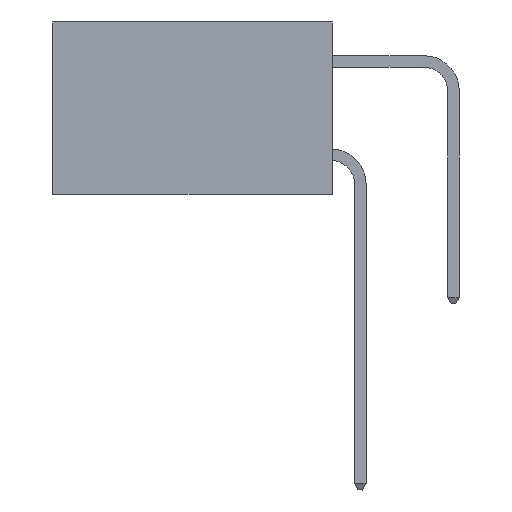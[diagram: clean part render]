
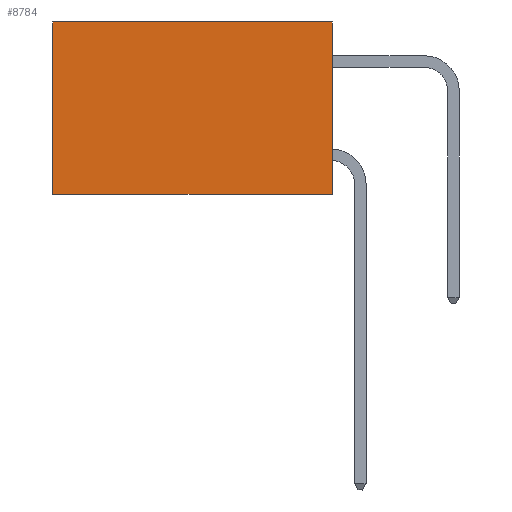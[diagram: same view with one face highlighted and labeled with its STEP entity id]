
A CAD part, left-side view. The second image highlights one B-rep face of the part: STEP entity #8784.
In plain terms, the highlighted planar face has unit normal (-1, 0, 0).
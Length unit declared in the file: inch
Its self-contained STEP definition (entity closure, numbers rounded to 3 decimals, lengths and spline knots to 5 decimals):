
#136 = FACE_OUTER_BOUND ( 'NONE', #17684, .T. ) ;
#1289 = VERTEX_POINT ( 'NONE', #6100 ) ;
#1593 = EDGE_CURVE ( 'NONE', #7111, #9854, #18074, .T. ) ;
#1920 = DIRECTION ( 'NONE',  ( 0., 1., 0. ) ) ;
#2348 = PLANE ( 'NONE',  #16039 ) ;
#2516 = EDGE_CURVE ( 'NONE', #5269, #1289, #4858, .T. ) ;
#4044 = CARTESIAN_POINT ( 'NONE',  ( 0.298, 0., -0.37 ) ) ;
#4463 = DIRECTION ( 'NONE',  ( 1., 0., 0. ) ) ;
#4858 = LINE ( 'NONE', #19780, #14758 ) ;
#4864 = CARTESIAN_POINT ( 'NONE',  ( 0.298, 0., 0. ) ) ;
#5269 = VERTEX_POINT ( 'NONE', #17595 ) ;
#6100 = CARTESIAN_POINT ( 'NONE',  ( 0.298, 0.6, 0. ) ) ;
#7111 = VERTEX_POINT ( 'NONE', #13817 ) ;
#7821 = VECTOR ( 'NONE', #18948, 39.37008 ) ;
#8350 = ORIENTED_EDGE ( 'NONE', *, *, #21593, .F. ) ;
#8784 = ADVANCED_FACE ( 'NONE', ( #136 ), #2348, .F. ) ;
#9854 = VERTEX_POINT ( 'NONE', #23760 ) ;
#12603 = EDGE_CURVE ( 'NONE', #1289, #9854, #21689, .T. ) ;
#13795 = VECTOR ( 'NONE', #1920, 39.37008 ) ;
#13817 = CARTESIAN_POINT ( 'NONE',  ( 0.298, 0., -0.37 ) ) ;
#14229 = ORIENTED_EDGE ( 'NONE', *, *, #2516, .T. ) ;
#14758 = VECTOR ( 'NONE', #23289, 39.37008 ) ;
#16039 = AXIS2_PLACEMENT_3D ( 'NONE', #22189, #4463, #20253 ) ;
#16860 = ORIENTED_EDGE ( 'NONE', *, *, #1593, .F. ) ;
#17594 = VECTOR ( 'NONE', #20561, 39.37008 ) ;
#17595 = CARTESIAN_POINT ( 'NONE',  ( 0.298, 0., 0. ) ) ;
#17684 = EDGE_LOOP ( 'NONE', ( #20352, #16860, #8350, #14229 ) ) ;
#18074 = LINE ( 'NONE', #4044, #13795 ) ;
#18948 = DIRECTION ( 'NONE',  ( 0., 0., -1. ) ) ;
#19780 = CARTESIAN_POINT ( 'NONE',  ( 0.298, 0., 0. ) ) ;
#20253 = DIRECTION ( 'NONE',  ( 0., 0., -1. ) ) ;
#20352 = ORIENTED_EDGE ( 'NONE', *, *, #12603, .T. ) ;
#20561 = DIRECTION ( 'NONE',  ( 0., 0., -1. ) ) ;
#21593 = EDGE_CURVE ( 'NONE', #5269, #7111, #22814, .T. ) ;
#21689 = LINE ( 'NONE', #23077, #7821 ) ;
#22189 = CARTESIAN_POINT ( 'NONE',  ( 0.298, 0., 0. ) ) ;
#22814 = LINE ( 'NONE', #4864, #17594 ) ;
#23077 = CARTESIAN_POINT ( 'NONE',  ( 0.298, 0.6, 0. ) ) ;
#23289 = DIRECTION ( 'NONE',  ( 0., 1., 0. ) ) ;
#23760 = CARTESIAN_POINT ( 'NONE',  ( 0.298, 0.6, -0.37 ) ) ;
